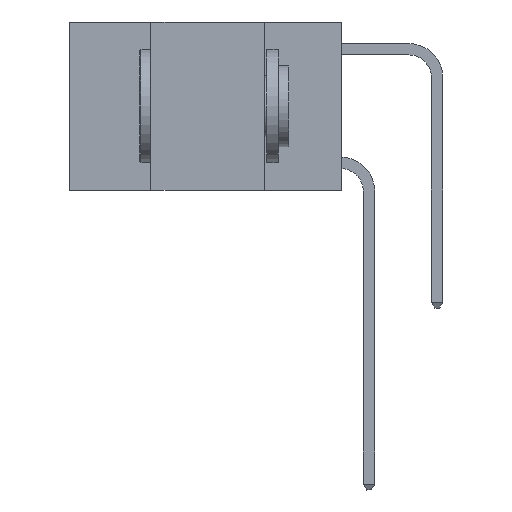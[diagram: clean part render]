
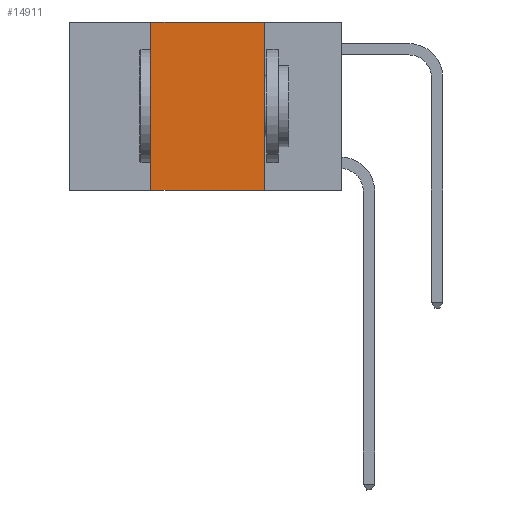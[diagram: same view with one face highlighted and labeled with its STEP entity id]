
A CAD part, left-side view. The second image highlights one B-rep face of the part: STEP entity #14911.
In plain terms, the highlighted planar face has unit normal (-1, 0, 0).
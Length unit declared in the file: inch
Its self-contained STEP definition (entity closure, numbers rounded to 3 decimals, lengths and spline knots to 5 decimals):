
#634 = EDGE_LOOP ( 'NONE', ( #3394, #10931, #9950, #10669 ) ) ;
#1955 = CARTESIAN_POINT ( 'NONE',  ( 0., 0.6, 0. ) ) ;
#2940 = CARTESIAN_POINT ( 'NONE',  ( 0., 0.6, 0. ) ) ;
#3197 = CARTESIAN_POINT ( 'NONE',  ( 0., 0.6, -0.37 ) ) ;
#3394 = ORIENTED_EDGE ( 'NONE', *, *, #10681, .F. ) ;
#4182 = EDGE_CURVE ( 'NONE', #11062, #12858, #15335, .T. ) ;
#5066 = EDGE_CURVE ( 'NONE', #10295, #10452, #14771, .T. ) ;
#5351 = CARTESIAN_POINT ( 'NONE',  ( 0., 0.42, 0. ) ) ;
#5568 = DIRECTION ( 'NONE',  ( 0., -1., 0. ) ) ;
#5572 = DIRECTION ( 'NONE',  ( 0., 0., -1. ) ) ;
#5604 = CARTESIAN_POINT ( 'NONE',  ( 0., 0.17, -0.37 ) ) ;
#5964 = AXIS2_PLACEMENT_3D ( 'NONE', #1955, #7889, #7940 ) ;
#7127 = CARTESIAN_POINT ( 'NONE',  ( 0., 0.42, 0. ) ) ;
#7702 = VECTOR ( 'NONE', #9102, 39.37008 ) ;
#7889 = DIRECTION ( 'NONE',  ( 1., 0., 0. ) ) ;
#7940 = DIRECTION ( 'NONE',  ( 0., 0., -1. ) ) ;
#9102 = DIRECTION ( 'NONE',  ( 0., 0., 1. ) ) ;
#9196 = VECTOR ( 'NONE', #5572, 39.37008 ) ;
#9950 = ORIENTED_EDGE ( 'NONE', *, *, #11505, .F. ) ;
#10141 = VECTOR ( 'NONE', #5568, 39.37008 ) ;
#10295 = VERTEX_POINT ( 'NONE', #5351 ) ;
#10452 = VERTEX_POINT ( 'NONE', #12139 ) ;
#10669 = ORIENTED_EDGE ( 'NONE', *, *, #4182, .T. ) ;
#10681 = EDGE_CURVE ( 'NONE', #10452, #12858, #11103, .T. ) ;
#10931 = ORIENTED_EDGE ( 'NONE', *, *, #5066, .F. ) ;
#10986 = CARTESIAN_POINT ( 'NONE',  ( 0., 0.42, -0.37 ) ) ;
#11062 = VERTEX_POINT ( 'NONE', #10986 ) ;
#11103 = LINE ( 'NONE', #15165, #9196 ) ;
#11502 = FACE_OUTER_BOUND ( 'NONE', #634, .T. ) ;
#11505 = EDGE_CURVE ( 'NONE', #11062, #10295, #14398, .T. ) ;
#12139 = CARTESIAN_POINT ( 'NONE',  ( 0., 0.17, 0. ) ) ;
#12858 = VERTEX_POINT ( 'NONE', #5604 ) ;
#13874 = DIRECTION ( 'NONE',  ( 0., -1., 0. ) ) ;
#14228 = VECTOR ( 'NONE', #13874, 39.37008 ) ;
#14398 = LINE ( 'NONE', #7127, #7702 ) ;
#14771 = LINE ( 'NONE', #2940, #14228 ) ;
#14911 = ADVANCED_FACE ( 'NONE', ( #11502 ), #15057, .F. ) ;
#15057 = PLANE ( 'NONE',  #5964 ) ;
#15165 = CARTESIAN_POINT ( 'NONE',  ( 0., 0.17, 0. ) ) ;
#15335 = LINE ( 'NONE', #3197, #10141 ) ;
